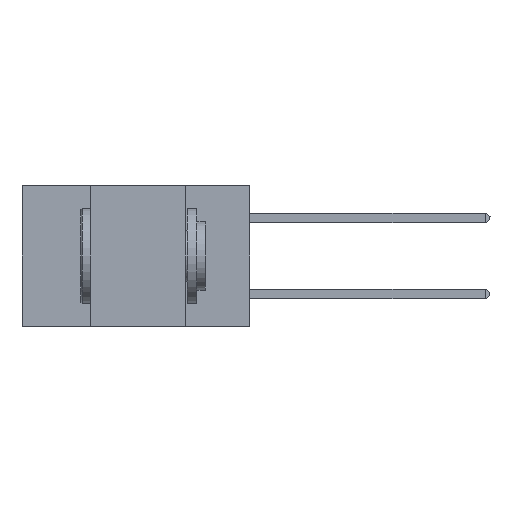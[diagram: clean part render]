
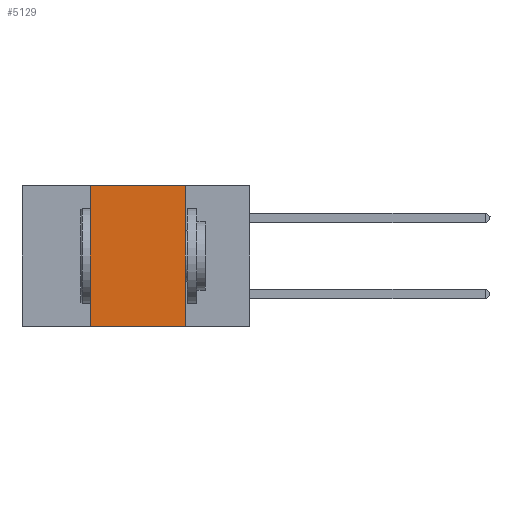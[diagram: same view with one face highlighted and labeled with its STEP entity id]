
A CAD part, left-side view. The second image highlights one B-rep face of the part: STEP entity #5129.
In plain terms, the highlighted planar face has unit normal (-1, 0, 0).
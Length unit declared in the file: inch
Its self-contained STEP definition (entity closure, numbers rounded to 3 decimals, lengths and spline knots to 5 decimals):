
#553 = LINE ( 'NONE', #17606, #25176 ) ;
#984 = ORIENTED_EDGE ( 'NONE', *, *, #26949, .F. ) ;
#1256 = DIRECTION ( 'NONE',  ( 0., 0., 1. ) ) ;
#1463 = ORIENTED_EDGE ( 'NONE', *, *, #19029, .F. ) ;
#1674 = ORIENTED_EDGE ( 'NONE', *, *, #26029, .F. ) ;
#1928 = VERTEX_POINT ( 'NONE', #22635 ) ;
#2520 = ORIENTED_EDGE ( 'NONE', *, *, #11164, .T. ) ;
#2568 = DIRECTION ( 'NONE',  ( 0., 0., -1. ) ) ;
#2880 = CARTESIAN_POINT ( 'NONE',  ( 0., 0.17, 0. ) ) ;
#2955 = CARTESIAN_POINT ( 'NONE',  ( 0., 0.42, 0. ) ) ;
#5129 = ADVANCED_FACE ( 'NONE', ( #28394 ), #19855, .F. ) ;
#5301 = CARTESIAN_POINT ( 'NONE',  ( 0., 0.6, -0.37 ) ) ;
#6081 = DIRECTION ( 'NONE',  ( 1., 0., 0. ) ) ;
#7754 = AXIS2_PLACEMENT_3D ( 'NONE', #26572, #6081, #22149 ) ;
#7953 = LINE ( 'NONE', #26805, #24716 ) ;
#8505 = DIRECTION ( 'NONE',  ( 0., -1., 0. ) ) ;
#10877 = VECTOR ( 'NONE', #2568, 39.37008 ) ;
#11164 = EDGE_CURVE ( 'NONE', #1928, #11228, #23985, .T. ) ;
#11189 = VERTEX_POINT ( 'NONE', #2955 ) ;
#11228 = VERTEX_POINT ( 'NONE', #28296 ) ;
#14489 = CARTESIAN_POINT ( 'NONE',  ( 0., 0.17, 0. ) ) ;
#17003 = LINE ( 'NONE', #14489, #10877 ) ;
#17606 = CARTESIAN_POINT ( 'NONE',  ( 0., 0.42, 0. ) ) ;
#17956 = VECTOR ( 'NONE', #19112, 39.37008 ) ;
#19029 = EDGE_CURVE ( 'NONE', #11189, #25161, #7953, .T. ) ;
#19112 = DIRECTION ( 'NONE',  ( 0., -1., 0. ) ) ;
#19855 = PLANE ( 'NONE',  #7754 ) ;
#19887 = EDGE_LOOP ( 'NONE', ( #984, #1463, #1674, #2520 ) ) ;
#22149 = DIRECTION ( 'NONE',  ( 0., 0., -1. ) ) ;
#22635 = CARTESIAN_POINT ( 'NONE',  ( 0., 0.42, -0.37 ) ) ;
#23985 = LINE ( 'NONE', #5301, #17956 ) ;
#24716 = VECTOR ( 'NONE', #8505, 39.37008 ) ;
#25161 = VERTEX_POINT ( 'NONE', #2880 ) ;
#25176 = VECTOR ( 'NONE', #1256, 39.37008 ) ;
#26029 = EDGE_CURVE ( 'NONE', #1928, #11189, #553, .T. ) ;
#26572 = CARTESIAN_POINT ( 'NONE',  ( 0., 0.6, 0. ) ) ;
#26805 = CARTESIAN_POINT ( 'NONE',  ( 0., 0.6, 0. ) ) ;
#26949 = EDGE_CURVE ( 'NONE', #25161, #11228, #17003, .T. ) ;
#28296 = CARTESIAN_POINT ( 'NONE',  ( 0., 0.17, -0.37 ) ) ;
#28394 = FACE_OUTER_BOUND ( 'NONE', #19887, .T. ) ;
